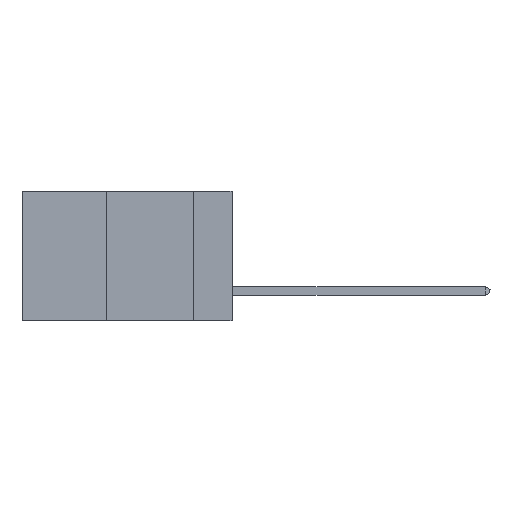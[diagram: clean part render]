
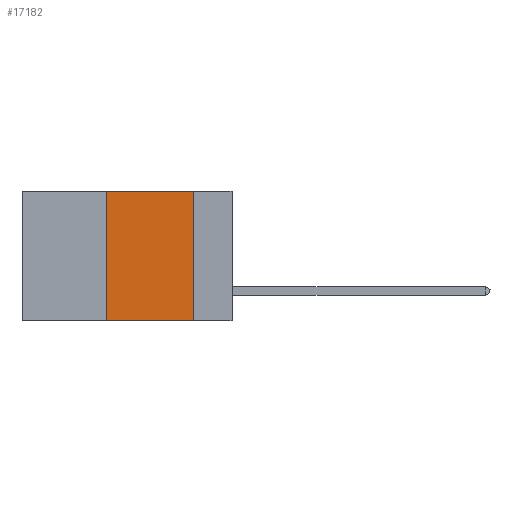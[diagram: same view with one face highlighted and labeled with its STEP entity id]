
A CAD part, left-side view. The second image highlights one B-rep face of the part: STEP entity #17182.
In plain terms, the highlighted planar face has unit normal (-1, 0, 0).
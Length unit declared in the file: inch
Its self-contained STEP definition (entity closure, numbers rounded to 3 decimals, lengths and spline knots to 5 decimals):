
#859 = FACE_OUTER_BOUND ( 'NONE', #11587, .T. ) ;
#2255 = VERTEX_POINT ( 'NONE', #25692 ) ;
#3544 = VERTEX_POINT ( 'NONE', #18603 ) ;
#4316 = VECTOR ( 'NONE', #33228, 39.37008 ) ;
#5814 = LINE ( 'NONE', #17186, #12512 ) ;
#8061 = CARTESIAN_POINT ( 'NONE',  ( 0., 0.11, 0. ) ) ;
#9227 = CARTESIAN_POINT ( 'NONE',  ( 0., 0.6, 0. ) ) ;
#9997 = CARTESIAN_POINT ( 'NONE',  ( 0., 0.11, -0.37 ) ) ;
#10956 = LINE ( 'NONE', #19179, #4316 ) ;
#11270 = DIRECTION ( 'NONE',  ( 0., 0., 1. ) ) ;
#11587 = EDGE_LOOP ( 'NONE', ( #17803, #18242, #13080, #39538 ) ) ;
#12512 = VECTOR ( 'NONE', #18107, 39.37008 ) ;
#12918 = PLANE ( 'NONE',  #34099 ) ;
#13080 = ORIENTED_EDGE ( 'NONE', *, *, #16914, .F. ) ;
#14712 = VERTEX_POINT ( 'NONE', #9997 ) ;
#16332 = DIRECTION ( 'NONE',  ( 0., -1., 0. ) ) ;
#16914 = EDGE_CURVE ( 'NONE', #2255, #3544, #28626, .T. ) ;
#17182 = ADVANCED_FACE ( 'NONE', ( #859 ), #12918, .F. ) ;
#17186 = CARTESIAN_POINT ( 'NONE',  ( 0., 0.6, -0.37 ) ) ;
#17803 = ORIENTED_EDGE ( 'NONE', *, *, #39029, .F. ) ;
#18107 = DIRECTION ( 'NONE',  ( 0., -1., 0. ) ) ;
#18242 = ORIENTED_EDGE ( 'NONE', *, *, #27188, .F. ) ;
#18603 = CARTESIAN_POINT ( 'NONE',  ( 0., 0.36, 0. ) ) ;
#19179 = CARTESIAN_POINT ( 'NONE',  ( 0., 0.11, 0. ) ) ;
#20081 = CARTESIAN_POINT ( 'NONE',  ( 0., 0.6, 0. ) ) ;
#20277 = VECTOR ( 'NONE', #11270, 39.37008 ) ;
#22872 = LINE ( 'NONE', #20081, #37377 ) ;
#23480 = DIRECTION ( 'NONE',  ( 1., 0., 0. ) ) ;
#25692 = CARTESIAN_POINT ( 'NONE',  ( 0., 0.36, -0.37 ) ) ;
#25872 = CARTESIAN_POINT ( 'NONE',  ( 0., 0.36, 0. ) ) ;
#27077 = DIRECTION ( 'NONE',  ( 0., 0., -1. ) ) ;
#27188 = EDGE_CURVE ( 'NONE', #3544, #38927, #22872, .T. ) ;
#28626 = LINE ( 'NONE', #25872, #20277 ) ;
#33228 = DIRECTION ( 'NONE',  ( 0., 0., -1. ) ) ;
#34099 = AXIS2_PLACEMENT_3D ( 'NONE', #9227, #23480, #27077 ) ;
#37377 = VECTOR ( 'NONE', #16332, 39.37008 ) ;
#38927 = VERTEX_POINT ( 'NONE', #8061 ) ;
#39029 = EDGE_CURVE ( 'NONE', #38927, #14712, #10956, .T. ) ;
#39538 = ORIENTED_EDGE ( 'NONE', *, *, #40589, .T. ) ;
#40589 = EDGE_CURVE ( 'NONE', #2255, #14712, #5814, .T. ) ;
